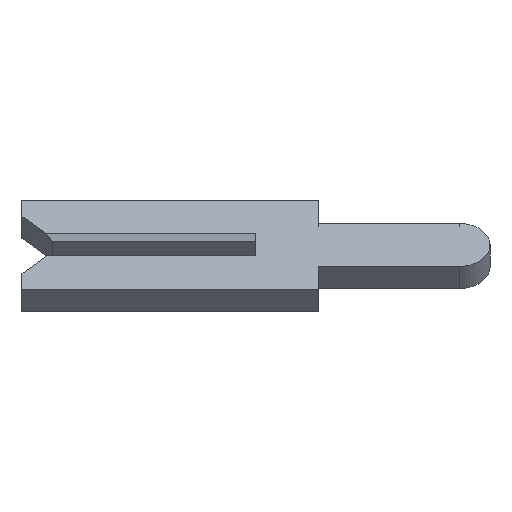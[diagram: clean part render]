
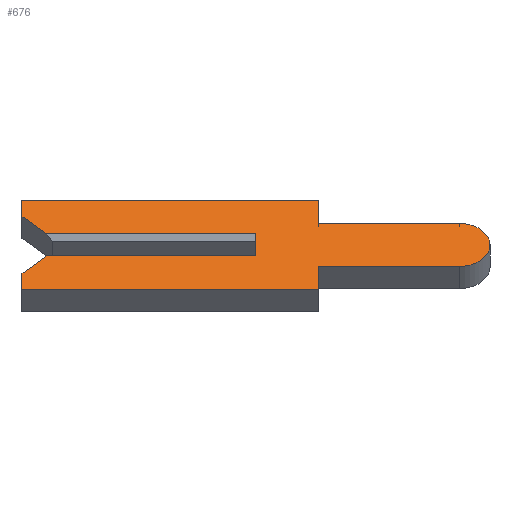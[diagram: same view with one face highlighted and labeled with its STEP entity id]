
A CAD part, left-side view. The second image highlights one B-rep face of the part: STEP entity #676.
In plain terms, the highlighted face is planar.
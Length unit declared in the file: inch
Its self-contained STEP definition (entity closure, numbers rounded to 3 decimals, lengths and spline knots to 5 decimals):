
#3 = EDGE_CURVE ( 'NONE', #490, #382, #357, .T. ) ;
#6 = VECTOR ( 'NONE', #400, 39.37008 ) ;
#12 = CARTESIAN_POINT ( 'NONE',  ( -0.01, 0.15, 0.026 ) ) ;
#26 = CARTESIAN_POINT ( 'NONE',  ( -0.01, -0.1305, -0.01 ) ) ;
#79 = CARTESIAN_POINT ( 'NONE',  ( -0.01, 0.15, -0.026 ) ) ;
#86 = CARTESIAN_POINT ( 'NONE',  ( -0.01, -0.1305, 0. ) ) ;
#101 = EDGE_CURVE ( 'NONE', #343, #278, #589, .T. ) ;
#113 = CARTESIAN_POINT ( 'NONE',  ( -0.01, 0.15, 0.026 ) ) ;
#117 = FACE_OUTER_BOUND ( 'NONE', #671, .T. ) ;
#128 = EDGE_CURVE ( 'NONE', #382, #466, #187, .T. ) ;
#132 = CARTESIAN_POINT ( 'NONE',  ( -0.01, 0., 0.01 ) ) ;
#137 = DIRECTION ( 'NONE',  ( 0., -1., 0. ) ) ;
#142 = VECTOR ( 'NONE', #613, 39.37008 ) ;
#158 = LINE ( 'NONE', #564, #1031 ) ;
#165 = EDGE_CURVE ( 'NONE', #741, #1107, #158, .T. ) ;
#168 = ORIENTED_EDGE ( 'NONE', *, *, #165, .F. ) ;
#187 = LINE ( 'NONE', #26, #142 ) ;
#203 = VECTOR ( 'NONE', #845, 39.37008 ) ;
#208 = VERTEX_POINT ( 'NONE', #132 ) ;
#218 = VECTOR ( 'NONE', #361, 39.37008 ) ;
#233 = LINE ( 'NONE', #612, #669 ) ;
#235 = DIRECTION ( 'NONE',  ( 0., 0., 1. ) ) ;
#237 = VERTEX_POINT ( 'NONE', #724 ) ;
#243 = DIRECTION ( 'NONE',  ( 0., 0., 1. ) ) ;
#247 = CARTESIAN_POINT ( 'NONE',  ( -0.01, 0.15, 0.04 ) ) ;
#265 = DIRECTION ( 'NONE',  ( 0., 0., -1. ) ) ;
#275 = CARTESIAN_POINT ( 'NONE',  ( -0.01, -0.04, -0.04 ) ) ;
#278 = VERTEX_POINT ( 'NONE', #657 ) ;
#282 = CARTESIAN_POINT ( 'NONE',  ( -0.01, 0.1305, 0.0065 ) ) ;
#299 = VECTOR ( 'NONE', #355, 39.37008 ) ;
#304 = ORIENTED_EDGE ( 'NONE', *, *, #440, .F. ) ;
#307 = ORIENTED_EDGE ( 'NONE', *, *, #565, .F. ) ;
#321 = CARTESIAN_POINT ( 'NONE',  ( -0.01, 0., 0.0065 ) ) ;
#330 = ORIENTED_EDGE ( 'NONE', *, *, #830, .F. ) ;
#342 = CIRCLE ( 'NONE', #682, 0.0195 ) ;
#343 = VERTEX_POINT ( 'NONE', #537 ) ;
#355 = DIRECTION ( 'NONE',  ( 0., 0., -1. ) ) ;
#357 = LINE ( 'NONE', #363, #851 ) ;
#359 = DIRECTION ( 'NONE',  ( 0., 0., -1. ) ) ;
#361 = DIRECTION ( 'NONE',  ( 0., 1., 0. ) ) ;
#363 = CARTESIAN_POINT ( 'NONE',  ( -0.01, 0.1305, -0.0065 ) ) ;
#373 = VERTEX_POINT ( 'NONE', #855 ) ;
#381 = EDGE_CURVE ( 'NONE', #683, #741, #1073, .T. ) ;
#382 = VERTEX_POINT ( 'NONE', #414 ) ;
#400 = DIRECTION ( 'NONE',  ( 0., 0., 1. ) ) ;
#410 = LINE ( 'NONE', #282, #782 ) ;
#414 = CARTESIAN_POINT ( 'NONE',  ( -0.01, 0.134, -0.01 ) ) ;
#425 = CARTESIAN_POINT ( 'NONE',  ( -0.01, -0.04, 0.0195 ) ) ;
#431 = LINE ( 'NONE', #321, #1062 ) ;
#437 = DIRECTION ( 'NONE',  ( 1., 0., 0. ) ) ;
#440 = EDGE_CURVE ( 'NONE', #568, #490, #522, .T. ) ;
#466 = VERTEX_POINT ( 'NONE', #1113 ) ;
#476 = ORIENTED_EDGE ( 'NONE', *, *, #507, .F. ) ;
#490 = VERTEX_POINT ( 'NONE', #668 ) ;
#491 = ORIENTED_EDGE ( 'NONE', *, *, #893, .T. ) ;
#493 = EDGE_CURVE ( 'NONE', #466, #208, #431, .T. ) ;
#507 = EDGE_CURVE ( 'NONE', #1107, #616, #793, .T. ) ;
#522 = LINE ( 'NONE', #79, #996 ) ;
#537 = CARTESIAN_POINT ( 'NONE',  ( -0.01, -0.04, -0.0195 ) ) ;
#545 = VECTOR ( 'NONE', #772, 39.37008 ) ;
#564 = CARTESIAN_POINT ( 'NONE',  ( -0.01, 0.15, 0.04 ) ) ;
#565 = EDGE_CURVE ( 'NONE', #616, #373, #847, .T. ) ;
#568 = VERTEX_POINT ( 'NONE', #945 ) ;
#571 = ORIENTED_EDGE ( 'NONE', *, *, #128, .F. ) ;
#585 = ORIENTED_EDGE ( 'NONE', *, *, #673, .F. ) ;
#589 = LINE ( 'NONE', #275, #299 ) ;
#598 = ORIENTED_EDGE ( 'NONE', *, *, #493, .F. ) ;
#600 = CARTESIAN_POINT ( 'NONE',  ( -0.01, -0.04, -0.0195 ) ) ;
#612 = CARTESIAN_POINT ( 'NONE',  ( -0.01, 0.15, 0.01 ) ) ;
#613 = DIRECTION ( 'NONE',  ( 0., -1., 0. ) ) ;
#616 = VERTEX_POINT ( 'NONE', #425 ) ;
#629 = VERTEX_POINT ( 'NONE', #970 ) ;
#657 = CARTESIAN_POINT ( 'NONE',  ( -0.01, -0.04, -0.04 ) ) ;
#668 = CARTESIAN_POINT ( 'NONE',  ( -0.01, 0.15, -0.026 ) ) ;
#669 = VECTOR ( 'NONE', #807, 39.37008 ) ;
#671 = EDGE_LOOP ( 'NONE', ( #491, #598, #571, #714, #304, #700, #765, #585, #330, #307, #476, #168, #1082, #927 ) ) ;
#673 = EDGE_CURVE ( 'NONE', #629, #343, #1032, .T. ) ;
#676 = ADVANCED_FACE ( 'NONE', ( #117 ), #957, .F. ) ;
#682 = AXIS2_PLACEMENT_3D ( 'NONE', #888, #437, #359 ) ;
#683 = VERTEX_POINT ( 'NONE', #12 ) ;
#700 = ORIENTED_EDGE ( 'NONE', *, *, #920, .F. ) ;
#714 = ORIENTED_EDGE ( 'NONE', *, *, #3, .F. ) ;
#723 = VECTOR ( 'NONE', #850, 39.37008 ) ;
#724 = CARTESIAN_POINT ( 'NONE',  ( -0.01, 0.134, 0.01 ) ) ;
#741 = VERTEX_POINT ( 'NONE', #247 ) ;
#757 = CARTESIAN_POINT ( 'NONE',  ( -0.01, -0.04, 0.0195 ) ) ;
#759 = CARTESIAN_POINT ( 'NONE',  ( -0.01, -0.04, 0.04 ) ) ;
#765 = ORIENTED_EDGE ( 'NONE', *, *, #101, .F. ) ;
#772 = DIRECTION ( 'NONE',  ( 0., 1., 0. ) ) ;
#782 = VECTOR ( 'NONE', #1079, 39.37008 ) ;
#793 = LINE ( 'NONE', #759, #203 ) ;
#807 = DIRECTION ( 'NONE',  ( 0., -1., 0. ) ) ;
#830 = EDGE_CURVE ( 'NONE', #373, #629, #342, .T. ) ;
#845 = DIRECTION ( 'NONE',  ( 0., 0., -1. ) ) ;
#847 = LINE ( 'NONE', #757, #723 ) ;
#850 = DIRECTION ( 'NONE',  ( 0., -1., 0. ) ) ;
#851 = VECTOR ( 'NONE', #877, 39.37008 ) ;
#855 = CARTESIAN_POINT ( 'NONE',  ( -0.01, -0.1305, 0.0195 ) ) ;
#877 = DIRECTION ( 'NONE',  ( 0., -0.707, 0.707 ) ) ;
#888 = CARTESIAN_POINT ( 'NONE',  ( -0.01, -0.1305, 0. ) ) ;
#893 = EDGE_CURVE ( 'NONE', #237, #208, #233, .T. ) ;
#914 = LINE ( 'NONE', #985, #218 ) ;
#917 = CARTESIAN_POINT ( 'NONE',  ( -0.01, -0.04, 0.04 ) ) ;
#920 = EDGE_CURVE ( 'NONE', #278, #568, #914, .T. ) ;
#927 = ORIENTED_EDGE ( 'NONE', *, *, #1077, .F. ) ;
#945 = CARTESIAN_POINT ( 'NONE',  ( -0.01, 0.15, -0.04 ) ) ;
#957 = PLANE ( 'NONE',  #1012 ) ;
#964 = DIRECTION ( 'NONE',  ( 1., 0., 0. ) ) ;
#970 = CARTESIAN_POINT ( 'NONE',  ( -0.01, -0.1305, -0.0195 ) ) ;
#985 = CARTESIAN_POINT ( 'NONE',  ( -0.01, 0.15, -0.04 ) ) ;
#996 = VECTOR ( 'NONE', #243, 39.37008 ) ;
#1012 = AXIS2_PLACEMENT_3D ( 'NONE', #86, #964, #265 ) ;
#1031 = VECTOR ( 'NONE', #137, 39.37008 ) ;
#1032 = LINE ( 'NONE', #600, #545 ) ;
#1062 = VECTOR ( 'NONE', #235, 39.37008 ) ;
#1073 = LINE ( 'NONE', #113, #6 ) ;
#1077 = EDGE_CURVE ( 'NONE', #237, #683, #410, .T. ) ;
#1079 = DIRECTION ( 'NONE',  ( 0., 0.707, 0.707 ) ) ;
#1082 = ORIENTED_EDGE ( 'NONE', *, *, #381, .F. ) ;
#1107 = VERTEX_POINT ( 'NONE', #917 ) ;
#1113 = CARTESIAN_POINT ( 'NONE',  ( -0.01, 0., -0.01 ) ) ;
